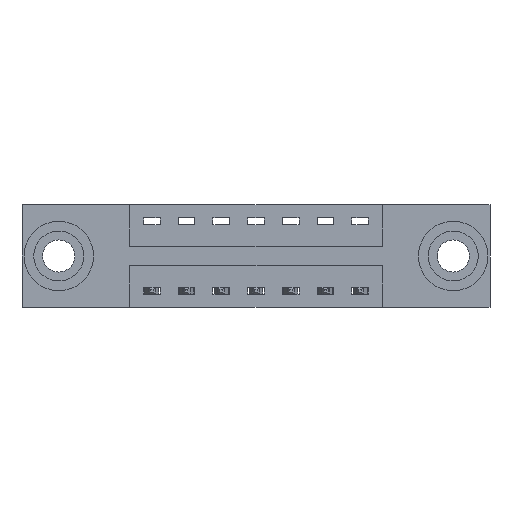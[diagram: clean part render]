
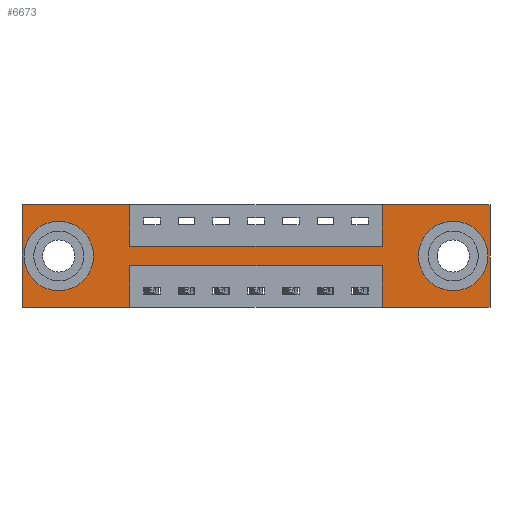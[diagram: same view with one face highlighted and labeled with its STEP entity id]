
A CAD part, front view. The second image highlights one B-rep face of the part: STEP entity #6673.
In plain terms, the highlighted planar face has unit normal (0, -1, 0).
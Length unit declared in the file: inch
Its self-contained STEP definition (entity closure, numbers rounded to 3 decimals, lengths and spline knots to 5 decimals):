
#434 = VERTEX_POINT ( 'NONE', #7800 ) ;
#489 = ORIENTED_EDGE ( 'NONE', *, *, #2340, .F. ) ;
#515 = DIRECTION ( 'NONE',  ( 0., 0., -1. ) ) ;
#541 = LINE ( 'NONE', #3882, #2540 ) ;
#552 = VERTEX_POINT ( 'NONE', #6682 ) ;
#623 = CARTESIAN_POINT ( 'NONE',  ( 0.3875, 0., -0.15 ) ) ;
#725 = CARTESIAN_POINT ( 'NONE',  ( 0.1325, 0., -0.263 ) ) ;
#727 = ORIENTED_EDGE ( 'NONE', *, *, #8723, .F. ) ;
#859 = VERTEX_POINT ( 'NONE', #8232 ) ;
#878 = VERTEX_POINT ( 'NONE', #6168 ) ;
#937 = EDGE_CURVE ( 'NONE', #878, #552, #1593, .T. ) ;
#1017 = EDGE_LOOP ( 'NONE', ( #7268, #3410, #727, #5242, #1942, #3081, #7366, #489, #1368, #3613, #4025, #9599 ) ) ;
#1368 = ORIENTED_EDGE ( 'NONE', *, *, #3305, .F. ) ;
#1397 = VERTEX_POINT ( 'NONE', #2968 ) ;
#1404 = LINE ( 'NONE', #1418, #6271 ) ;
#1408 = AXIS2_PLACEMENT_3D ( 'NONE', #5329, #8977, #515 ) ;
#1418 = CARTESIAN_POINT ( 'NONE',  ( 0.3875, 0., -0.37 ) ) ;
#1488 = AXIS2_PLACEMENT_3D ( 'NONE', #4985, #8578, #2689 ) ;
#1525 = VERTEX_POINT ( 'NONE', #8450 ) ;
#1593 = LINE ( 'NONE', #7314, #5544 ) ;
#1605 = DIRECTION ( 'NONE',  ( -1., 0., 0. ) ) ;
#1650 = VERTEX_POINT ( 'NONE', #5477 ) ;
#1660 = DIRECTION ( 'NONE',  ( 0., 1., 0. ) ) ;
#1809 = VERTEX_POINT ( 'NONE', #3628 ) ;
#1926 = EDGE_CURVE ( 'NONE', #1397, #5073, #3024, .T. ) ;
#1942 = ORIENTED_EDGE ( 'NONE', *, *, #8542, .F. ) ;
#1971 = CARTESIAN_POINT ( 'NONE',  ( 0., 0., -0.37 ) ) ;
#2234 = DIRECTION ( 'NONE',  ( 0., 0., -1. ) ) ;
#2273 = VECTOR ( 'NONE', #3077, 39.37008 ) ;
#2340 = EDGE_CURVE ( 'NONE', #8700, #859, #5032, .T. ) ;
#2464 = CARTESIAN_POINT ( 'NONE',  ( 0.1325, 0., -0.185 ) ) ;
#2534 = CARTESIAN_POINT ( 'NONE',  ( 1.2975, 0., 0. ) ) ;
#2540 = VECTOR ( 'NONE', #4691, 39.37008 ) ;
#2599 = DIRECTION ( 'NONE',  ( 0., 1., 0. ) ) ;
#2649 = CARTESIAN_POINT ( 'NONE',  ( 0.3875, 0., -0.15 ) ) ;
#2689 = DIRECTION ( 'NONE',  ( 0., 0., 1. ) ) ;
#2715 = VECTOR ( 'NONE', #8912, 39.37008 ) ;
#2881 = EDGE_LOOP ( 'NONE', ( #9340, #6010 ) ) ;
#2968 = CARTESIAN_POINT ( 'NONE',  ( 1.5525, 0., -0.263 ) ) ;
#3003 = VECTOR ( 'NONE', #2234, 39.37008 ) ;
#3018 = CARTESIAN_POINT ( 'NONE',  ( 0., 0., -0.37 ) ) ;
#3024 = CIRCLE ( 'NONE', #9140, 0.078 ) ;
#3025 = VECTOR ( 'NONE', #3599, 39.37008 ) ;
#3077 = DIRECTION ( 'NONE',  ( -1., 0., 0. ) ) ;
#3081 = ORIENTED_EDGE ( 'NONE', *, *, #3889, .F. ) ;
#3305 = EDGE_CURVE ( 'NONE', #9415, #8700, #6435, .T. ) ;
#3410 = ORIENTED_EDGE ( 'NONE', *, *, #937, .F. ) ;
#3424 = CARTESIAN_POINT ( 'NONE',  ( 0.3875, 0., 0. ) ) ;
#3515 = LINE ( 'NONE', #3018, #3744 ) ;
#3599 = DIRECTION ( 'NONE',  ( 1., 0., 0. ) ) ;
#3613 = ORIENTED_EDGE ( 'NONE', *, *, #7310, .F. ) ;
#3628 = CARTESIAN_POINT ( 'NONE',  ( 0.1325, 0., -0.107 ) ) ;
#3726 = EDGE_CURVE ( 'NONE', #1650, #5963, #6527, .T. ) ;
#3744 = VECTOR ( 'NONE', #1605, 39.37008 ) ;
#3805 = CARTESIAN_POINT ( 'NONE',  ( 0., 0., -0.37 ) ) ;
#3879 = EDGE_CURVE ( 'NONE', #859, #8206, #5125, .T. ) ;
#3882 = CARTESIAN_POINT ( 'NONE',  ( 1.685, 0., 0. ) ) ;
#3889 = EDGE_CURVE ( 'NONE', #8206, #1525, #6867, .T. ) ;
#3908 = VECTOR ( 'NONE', #5693, 39.37008 ) ;
#4025 = ORIENTED_EDGE ( 'NONE', *, *, #5970, .F. ) ;
#4096 = FACE_BOUND ( 'NONE', #4954, .T. ) ;
#4170 = CIRCLE ( 'NONE', #6706, 0.078 ) ;
#4223 = DIRECTION ( 'NONE',  ( 0., 0., 1. ) ) ;
#4452 = LINE ( 'NONE', #6045, #6245 ) ;
#4691 = DIRECTION ( 'NONE',  ( 0., 0., -1. ) ) ;
#4703 = LINE ( 'NONE', #8111, #2715 ) ;
#4954 = EDGE_LOOP ( 'NONE', ( #8991, #6741 ) ) ;
#4985 = CARTESIAN_POINT ( 'NONE',  ( 0.1325, 0., -0.185 ) ) ;
#5032 = LINE ( 'NONE', #623, #3025 ) ;
#5073 = VERTEX_POINT ( 'NONE', #6663 ) ;
#5125 = LINE ( 'NONE', #7089, #3908 ) ;
#5242 = ORIENTED_EDGE ( 'NONE', *, *, #6219, .F. ) ;
#5329 = CARTESIAN_POINT ( 'NONE',  ( 1.5525, 0., -0.185 ) ) ;
#5477 = CARTESIAN_POINT ( 'NONE',  ( 0.3875, 0., -0.37 ) ) ;
#5541 = EDGE_CURVE ( 'NONE', #552, #1650, #1404, .T. ) ;
#5544 = VECTOR ( 'NONE', #8888, 39.37008 ) ;
#5693 = DIRECTION ( 'NONE',  ( 0., 0., 1. ) ) ;
#5792 = DIRECTION ( 'NONE',  ( 0., 0., -1. ) ) ;
#5954 = DIRECTION ( 'NONE',  ( 1., 0., 0. ) ) ;
#5963 = VERTEX_POINT ( 'NONE', #1971 ) ;
#5970 = EDGE_CURVE ( 'NONE', #5963, #434, #4703, .T. ) ;
#6004 = AXIS2_PLACEMENT_3D ( 'NONE', #3805, #6773, #9001 ) ;
#6010 = ORIENTED_EDGE ( 'NONE', *, *, #7798, .T. ) ;
#6045 = CARTESIAN_POINT ( 'NONE',  ( 0., 0., 0. ) ) ;
#6083 = CIRCLE ( 'NONE', #1408, 0.078 ) ;
#6109 = VECTOR ( 'NONE', #4223, 39.37008 ) ;
#6168 = CARTESIAN_POINT ( 'NONE',  ( 1.2975, 0., -0.22 ) ) ;
#6219 = EDGE_CURVE ( 'NONE', #7345, #8544, #3515, .T. ) ;
#6245 = VECTOR ( 'NONE', #5954, 39.37008 ) ;
#6271 = VECTOR ( 'NONE', #6694, 39.37008 ) ;
#6279 = DIRECTION ( 'NONE',  ( 0., 0., 1. ) ) ;
#6370 = CARTESIAN_POINT ( 'NONE',  ( 1.5525, 0., -0.185 ) ) ;
#6435 = LINE ( 'NONE', #3424, #3003 ) ;
#6527 = LINE ( 'NONE', #8761, #2273 ) ;
#6535 = CARTESIAN_POINT ( 'NONE',  ( 1.2975, 0., -0.37 ) ) ;
#6629 = CARTESIAN_POINT ( 'NONE',  ( 0., 0., 0. ) ) ;
#6663 = CARTESIAN_POINT ( 'NONE',  ( 1.5525, 0., -0.107 ) ) ;
#6673 = ADVANCED_FACE ( 'NONE', ( #4096, #7131, #8174 ), #8281, .T. ) ;
#6682 = CARTESIAN_POINT ( 'NONE',  ( 0.3875, 0., -0.22 ) ) ;
#6694 = DIRECTION ( 'NONE',  ( 0., 0., -1. ) ) ;
#6706 = AXIS2_PLACEMENT_3D ( 'NONE', #2464, #1660, #6279 ) ;
#6741 = ORIENTED_EDGE ( 'NONE', *, *, #1926, .T. ) ;
#6773 = DIRECTION ( 'NONE',  ( 0., -1., 0. ) ) ;
#6825 = CARTESIAN_POINT ( 'NONE',  ( 1.2975, 0., -0.37 ) ) ;
#6867 = LINE ( 'NONE', #6629, #9681 ) ;
#7089 = CARTESIAN_POINT ( 'NONE',  ( 1.2975, 0., 0. ) ) ;
#7131 = FACE_BOUND ( 'NONE', #2881, .T. ) ;
#7268 = ORIENTED_EDGE ( 'NONE', *, *, #5541, .F. ) ;
#7302 = CARTESIAN_POINT ( 'NONE',  ( 0.3875, 0., 0. ) ) ;
#7310 = EDGE_CURVE ( 'NONE', #434, #9415, #4452, .T. ) ;
#7314 = CARTESIAN_POINT ( 'NONE',  ( 0.3875, 0., -0.22 ) ) ;
#7345 = VERTEX_POINT ( 'NONE', #8170 ) ;
#7366 = ORIENTED_EDGE ( 'NONE', *, *, #3879, .F. ) ;
#7456 = DIRECTION ( 'NONE',  ( 1., 0., 0. ) ) ;
#7798 = EDGE_CURVE ( 'NONE', #9109, #1809, #9727, .T. ) ;
#7800 = CARTESIAN_POINT ( 'NONE',  ( 0., 0., 0. ) ) ;
#8111 = CARTESIAN_POINT ( 'NONE',  ( 0., 0., 0. ) ) ;
#8170 = CARTESIAN_POINT ( 'NONE',  ( 1.685, 0., -0.37 ) ) ;
#8174 = FACE_OUTER_BOUND ( 'NONE', #1017, .T. ) ;
#8206 = VERTEX_POINT ( 'NONE', #2534 ) ;
#8232 = CARTESIAN_POINT ( 'NONE',  ( 1.2975, 0., -0.15 ) ) ;
#8281 = PLANE ( 'NONE',  #6004 ) ;
#8450 = CARTESIAN_POINT ( 'NONE',  ( 1.685, 0., 0. ) ) ;
#8542 = EDGE_CURVE ( 'NONE', #1525, #7345, #541, .T. ) ;
#8544 = VERTEX_POINT ( 'NONE', #6825 ) ;
#8578 = DIRECTION ( 'NONE',  ( 0., 1., 0. ) ) ;
#8700 = VERTEX_POINT ( 'NONE', #2649 ) ;
#8723 = EDGE_CURVE ( 'NONE', #8544, #878, #8866, .T. ) ;
#8761 = CARTESIAN_POINT ( 'NONE',  ( 0., 0., -0.37 ) ) ;
#8866 = LINE ( 'NONE', #6535, #6109 ) ;
#8888 = DIRECTION ( 'NONE',  ( -1., 0., 0. ) ) ;
#8912 = DIRECTION ( 'NONE',  ( 0., 0., 1. ) ) ;
#8977 = DIRECTION ( 'NONE',  ( 0., 1., 0. ) ) ;
#8991 = ORIENTED_EDGE ( 'NONE', *, *, #9730, .T. ) ;
#9001 = DIRECTION ( 'NONE',  ( 0., 0., -1. ) ) ;
#9109 = VERTEX_POINT ( 'NONE', #725 ) ;
#9131 = EDGE_CURVE ( 'NONE', #1809, #9109, #4170, .T. ) ;
#9140 = AXIS2_PLACEMENT_3D ( 'NONE', #6370, #2599, #5792 ) ;
#9340 = ORIENTED_EDGE ( 'NONE', *, *, #9131, .T. ) ;
#9415 = VERTEX_POINT ( 'NONE', #7302 ) ;
#9599 = ORIENTED_EDGE ( 'NONE', *, *, #3726, .F. ) ;
#9681 = VECTOR ( 'NONE', #7456, 39.37008 ) ;
#9727 = CIRCLE ( 'NONE', #1488, 0.078 ) ;
#9730 = EDGE_CURVE ( 'NONE', #5073, #1397, #6083, .T. ) ;
